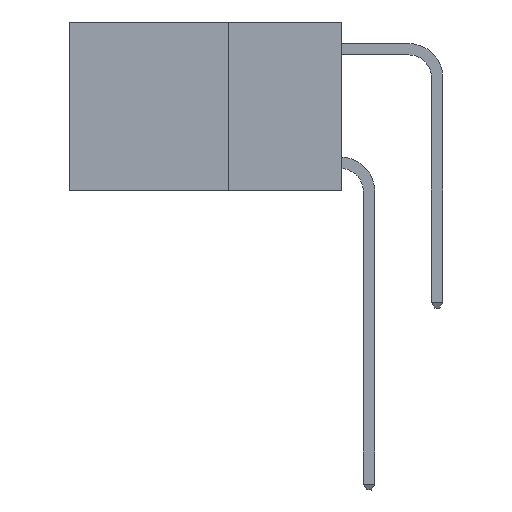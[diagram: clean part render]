
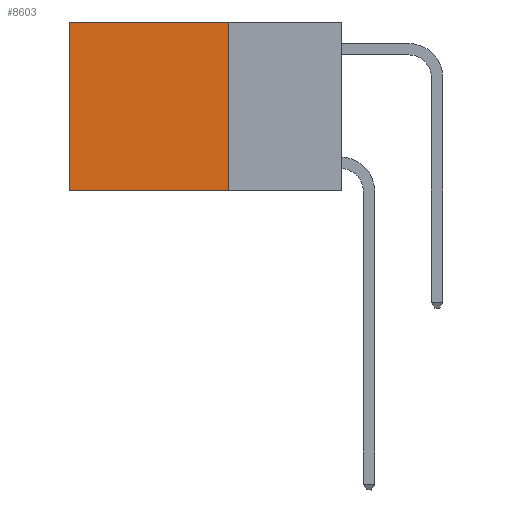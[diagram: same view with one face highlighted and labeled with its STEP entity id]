
A CAD part, left-side view. The second image highlights one B-rep face of the part: STEP entity #8603.
In plain terms, the highlighted planar face has unit normal (-1, 0, 0).
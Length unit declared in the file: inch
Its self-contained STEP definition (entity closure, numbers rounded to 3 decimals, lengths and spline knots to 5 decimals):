
#254 = VERTEX_POINT ( 'NONE', #11111 ) ;
#403 = VERTEX_POINT ( 'NONE', #9480 ) ;
#1760 = VERTEX_POINT ( 'NONE', #10868 ) ;
#1996 = LINE ( 'NONE', #13684, #7324 ) ;
#2427 = FACE_OUTER_BOUND ( 'NONE', #11945, .T. ) ;
#2703 = DIRECTION ( 'NONE',  ( 0., 0., -1. ) ) ;
#2933 = EDGE_CURVE ( 'NONE', #1760, #6143, #11459, .T. ) ;
#3228 = PLANE ( 'NONE',  #4023 ) ;
#3333 = EDGE_CURVE ( 'NONE', #403, #254, #5722, .T. ) ;
#3510 = VECTOR ( 'NONE', #12111, 39.37008 ) ;
#4023 = AXIS2_PLACEMENT_3D ( 'NONE', #8525, #5338, #12796 ) ;
#4628 = CARTESIAN_POINT ( 'NONE',  ( 0.2625, 0.25, -0.37 ) ) ;
#5338 = DIRECTION ( 'NONE',  ( 1., 0., 0. ) ) ;
#5651 = ORIENTED_EDGE ( 'NONE', *, *, #3333, .T. ) ;
#5722 = LINE ( 'NONE', #11870, #8253 ) ;
#5989 = ORIENTED_EDGE ( 'NONE', *, *, #2933, .F. ) ;
#6143 = VERTEX_POINT ( 'NONE', #10834 ) ;
#6312 = LINE ( 'NONE', #4628, #3510 ) ;
#6521 = DIRECTION ( 'NONE',  ( 0., 0., -1. ) ) ;
#7324 = VECTOR ( 'NONE', #12691, 39.37008 ) ;
#8253 = VECTOR ( 'NONE', #6521, 39.37008 ) ;
#8525 = CARTESIAN_POINT ( 'NONE',  ( 0.2625, 0.25, 0. ) ) ;
#8603 = ADVANCED_FACE ( 'NONE', ( #2427 ), #3228, .F. ) ;
#8845 = ORIENTED_EDGE ( 'NONE', *, *, #13616, .T. ) ;
#9480 = CARTESIAN_POINT ( 'NONE',  ( 0.2625, 0.6, 0. ) ) ;
#10834 = CARTESIAN_POINT ( 'NONE',  ( 0.2625, 0.25, -0.37 ) ) ;
#10868 = CARTESIAN_POINT ( 'NONE',  ( 0.2625, 0.25, 0. ) ) ;
#11111 = CARTESIAN_POINT ( 'NONE',  ( 0.2625, 0.6, -0.37 ) ) ;
#11239 = CARTESIAN_POINT ( 'NONE',  ( 0.2625, 0.25, 0. ) ) ;
#11378 = ORIENTED_EDGE ( 'NONE', *, *, #11479, .F. ) ;
#11459 = LINE ( 'NONE', #11239, #13559 ) ;
#11479 = EDGE_CURVE ( 'NONE', #6143, #254, #6312, .T. ) ;
#11870 = CARTESIAN_POINT ( 'NONE',  ( 0.2625, 0.6, 0. ) ) ;
#11945 = EDGE_LOOP ( 'NONE', ( #5651, #11378, #5989, #8845 ) ) ;
#12111 = DIRECTION ( 'NONE',  ( 0., 1., 0. ) ) ;
#12691 = DIRECTION ( 'NONE',  ( 0., 1., 0. ) ) ;
#12796 = DIRECTION ( 'NONE',  ( 0., 0., -1. ) ) ;
#13559 = VECTOR ( 'NONE', #2703, 39.37008 ) ;
#13616 = EDGE_CURVE ( 'NONE', #1760, #403, #1996, .T. ) ;
#13684 = CARTESIAN_POINT ( 'NONE',  ( 0.2625, 0.25, 0. ) ) ;
